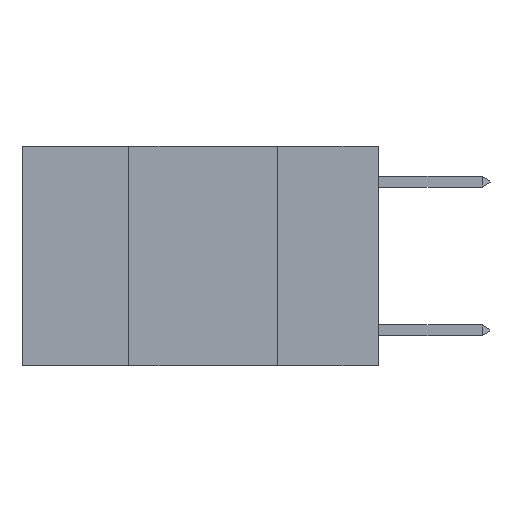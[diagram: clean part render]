
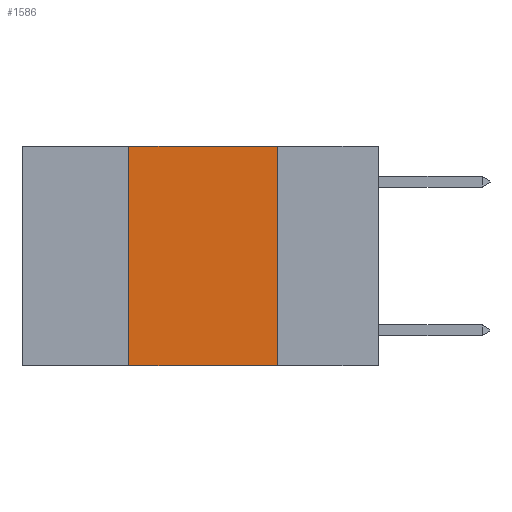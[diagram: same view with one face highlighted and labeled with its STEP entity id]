
A CAD part, left-side view. The second image highlights one B-rep face of the part: STEP entity #1586.
In plain terms, the highlighted planar face has unit normal (-1, 0, 0).
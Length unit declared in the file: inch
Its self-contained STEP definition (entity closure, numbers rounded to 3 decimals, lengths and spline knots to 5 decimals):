
#220 = VECTOR ( 'NONE', #8325, 39.37008 ) ;
#226 = LINE ( 'NONE', #8485, #220 ) ;
#690 = ORIENTED_EDGE ( 'NONE', *, *, #4178, .T. ) ;
#863 = CARTESIAN_POINT ( 'NONE',  ( 0., 0.42, 0. ) ) ;
#1014 = ORIENTED_EDGE ( 'NONE', *, *, #3122, .F. ) ;
#1586 = ADVANCED_FACE ( 'NONE', ( #3095 ), #2680, .F. ) ;
#2413 = EDGE_LOOP ( 'NONE', ( #7952, #1014, #7314, #690 ) ) ;
#2544 = DIRECTION ( 'NONE',  ( 0., 0., -1. ) ) ;
#2680 = PLANE ( 'NONE',  #3979 ) ;
#2778 = CARTESIAN_POINT ( 'NONE',  ( 0., 0.6, 0. ) ) ;
#3095 = FACE_OUTER_BOUND ( 'NONE', #2413, .T. ) ;
#3122 = EDGE_CURVE ( 'NONE', #5025, #6895, #4545, .T. ) ;
#3488 = VERTEX_POINT ( 'NONE', #5253 ) ;
#3861 = DIRECTION ( 'NONE',  ( 0., -1., 0. ) ) ;
#3909 = CARTESIAN_POINT ( 'NONE',  ( 0., 0.6, 0. ) ) ;
#3979 = AXIS2_PLACEMENT_3D ( 'NONE', #2778, #5766, #2544 ) ;
#4012 = EDGE_CURVE ( 'NONE', #6895, #3488, #226, .T. ) ;
#4178 = EDGE_CURVE ( 'NONE', #5465, #3488, #8062, .T. ) ;
#4204 = EDGE_CURVE ( 'NONE', #5465, #5025, #7861, .T. ) ;
#4526 = VECTOR ( 'NONE', #3861, 39.37008 ) ;
#4545 = LINE ( 'NONE', #3909, #4526 ) ;
#5025 = VERTEX_POINT ( 'NONE', #863 ) ;
#5244 = CARTESIAN_POINT ( 'NONE',  ( 0., 0.42, -0.37 ) ) ;
#5253 = CARTESIAN_POINT ( 'NONE',  ( 0., 0.17, -0.37 ) ) ;
#5383 = CARTESIAN_POINT ( 'NONE',  ( 0., 0.17, 0. ) ) ;
#5465 = VERTEX_POINT ( 'NONE', #5244 ) ;
#5766 = DIRECTION ( 'NONE',  ( 1., 0., 0. ) ) ;
#6895 = VERTEX_POINT ( 'NONE', #5383 ) ;
#7314 = ORIENTED_EDGE ( 'NONE', *, *, #4204, .F. ) ;
#7361 = DIRECTION ( 'NONE',  ( 0., 0., 1. ) ) ;
#7383 = CARTESIAN_POINT ( 'NONE',  ( 0., 0.42, 0. ) ) ;
#7441 = DIRECTION ( 'NONE',  ( 0., -1., 0. ) ) ;
#7499 = CARTESIAN_POINT ( 'NONE',  ( 0., 0.6, -0.37 ) ) ;
#7822 = VECTOR ( 'NONE', #7361, 39.37008 ) ;
#7861 = LINE ( 'NONE', #7383, #7822 ) ;
#7918 = VECTOR ( 'NONE', #7441, 39.37008 ) ;
#7952 = ORIENTED_EDGE ( 'NONE', *, *, #4012, .F. ) ;
#8062 = LINE ( 'NONE', #7499, #7918 ) ;
#8325 = DIRECTION ( 'NONE',  ( 0., 0., -1. ) ) ;
#8485 = CARTESIAN_POINT ( 'NONE',  ( 0., 0.17, 0. ) ) ;
